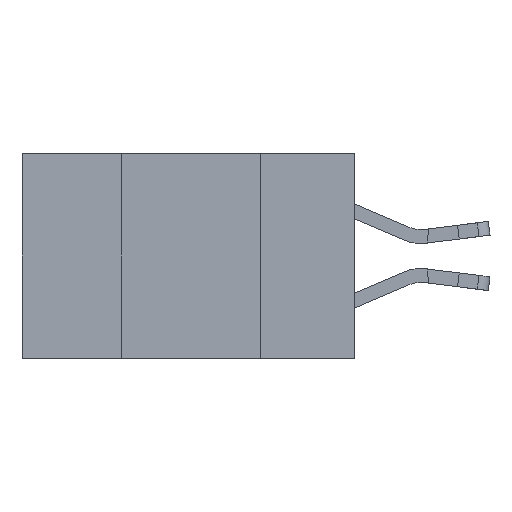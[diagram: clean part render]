
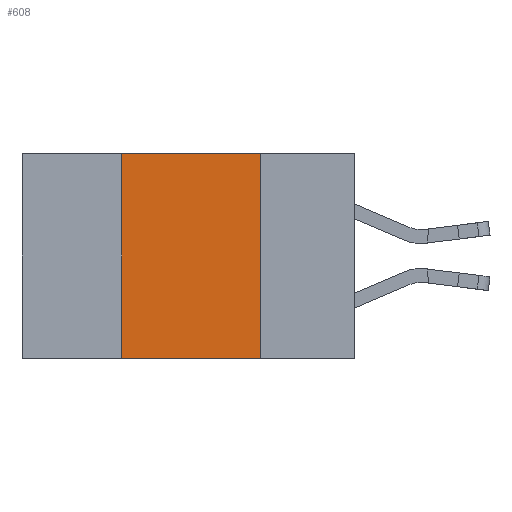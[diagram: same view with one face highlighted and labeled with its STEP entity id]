
A CAD part, left-side view. The second image highlights one B-rep face of the part: STEP entity #608.
In plain terms, the highlighted planar face has unit normal (-1, 0, 0).
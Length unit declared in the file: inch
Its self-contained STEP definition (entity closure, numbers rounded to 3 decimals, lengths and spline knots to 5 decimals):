
#608 = ADVANCED_FACE ( 'NONE', ( #11245 ), #4943, .F. ) ;
#1687 = DIRECTION ( 'NONE',  ( 0., -1., 0. ) ) ;
#2053 = VERTEX_POINT ( 'NONE', #4804 ) ;
#2178 = DIRECTION ( 'NONE',  ( 0., 0., -1. ) ) ;
#2495 = CARTESIAN_POINT ( 'NONE',  ( 0., 0.17, 0. ) ) ;
#2625 = EDGE_CURVE ( 'NONE', #10810, #8829, #10360, .T. ) ;
#2820 = VECTOR ( 'NONE', #2178, 39.37008 ) ;
#3310 = ORIENTED_EDGE ( 'NONE', *, *, #3861, .F. ) ;
#3861 = EDGE_CURVE ( 'NONE', #2053, #7405, #8956, .T. ) ;
#3976 = VECTOR ( 'NONE', #10893, 39.37008 ) ;
#4501 = CARTESIAN_POINT ( 'NONE',  ( 0., 0.17, 0. ) ) ;
#4631 = ORIENTED_EDGE ( 'NONE', *, *, #11718, .F. ) ;
#4804 = CARTESIAN_POINT ( 'NONE',  ( 0., 0.42, -0.37 ) ) ;
#4832 = CARTESIAN_POINT ( 'NONE',  ( 0., 0.42, 0. ) ) ;
#4943 = PLANE ( 'NONE',  #10956 ) ;
#5639 = ORIENTED_EDGE ( 'NONE', *, *, #5875, .T. ) ;
#5869 = EDGE_LOOP ( 'NONE', ( #7875, #4631, #3310, #5639 ) ) ;
#5875 = EDGE_CURVE ( 'NONE', #2053, #8829, #10909, .T. ) ;
#6438 = CARTESIAN_POINT ( 'NONE',  ( 0., 0.6, 0. ) ) ;
#6774 = DIRECTION ( 'NONE',  ( 0., -1., 0. ) ) ;
#6856 = DIRECTION ( 'NONE',  ( 1., 0., 0. ) ) ;
#7349 = LINE ( 'NONE', #12080, #9676 ) ;
#7405 = VERTEX_POINT ( 'NONE', #8010 ) ;
#7875 = ORIENTED_EDGE ( 'NONE', *, *, #2625, .F. ) ;
#8010 = CARTESIAN_POINT ( 'NONE',  ( 0., 0.42, 0. ) ) ;
#8573 = VECTOR ( 'NONE', #1687, 39.37008 ) ;
#8829 = VERTEX_POINT ( 'NONE', #10694 ) ;
#8956 = LINE ( 'NONE', #4832, #3976 ) ;
#9676 = VECTOR ( 'NONE', #6774, 39.37008 ) ;
#9815 = DIRECTION ( 'NONE',  ( 0., 0., -1. ) ) ;
#9956 = CARTESIAN_POINT ( 'NONE',  ( 0., 0.6, -0.37 ) ) ;
#10360 = LINE ( 'NONE', #2495, #2820 ) ;
#10694 = CARTESIAN_POINT ( 'NONE',  ( 0., 0.17, -0.37 ) ) ;
#10810 = VERTEX_POINT ( 'NONE', #4501 ) ;
#10893 = DIRECTION ( 'NONE',  ( 0., 0., 1. ) ) ;
#10909 = LINE ( 'NONE', #9956, #8573 ) ;
#10956 = AXIS2_PLACEMENT_3D ( 'NONE', #6438, #6856, #9815 ) ;
#11245 = FACE_OUTER_BOUND ( 'NONE', #5869, .T. ) ;
#11718 = EDGE_CURVE ( 'NONE', #7405, #10810, #7349, .T. ) ;
#12080 = CARTESIAN_POINT ( 'NONE',  ( 0., 0.6, 0. ) ) ;
